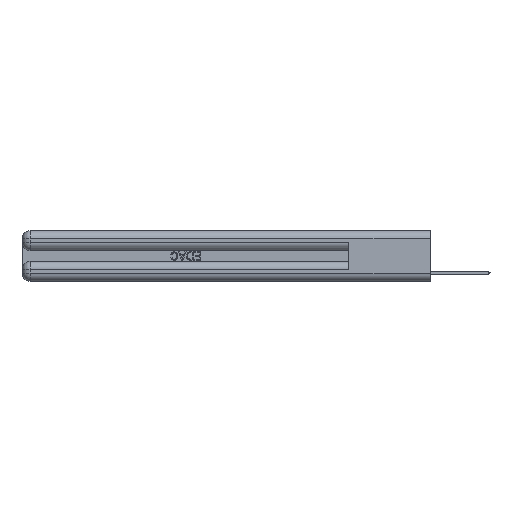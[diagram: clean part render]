
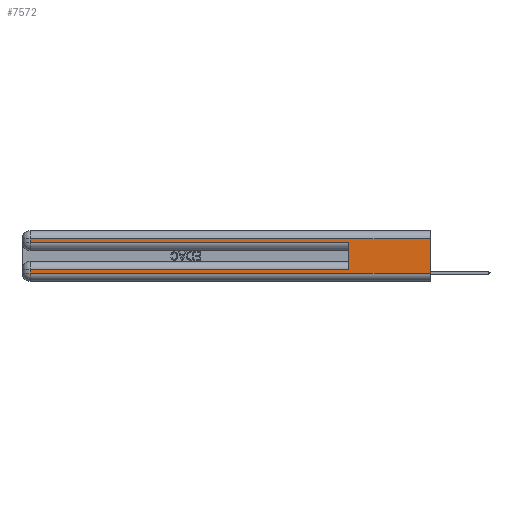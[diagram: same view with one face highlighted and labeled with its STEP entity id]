
A CAD part, left-side view. The second image highlights one B-rep face of the part: STEP entity #7572.
In plain terms, the highlighted planar face has unit normal (-1, 0, 0).
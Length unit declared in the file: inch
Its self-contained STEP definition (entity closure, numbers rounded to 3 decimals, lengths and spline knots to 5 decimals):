
#31 = CARTESIAN_POINT ( 'NONE',  ( 0., 2.94, 0.285 ) ) ;
#179 = CARTESIAN_POINT ( 'NONE',  ( 0., 2.94, 0.06 ) ) ;
#347 = VECTOR ( 'NONE', #25590, 39.37008 ) ;
#1287 = VERTEX_POINT ( 'NONE', #4405 ) ;
#1379 = ORIENTED_EDGE ( 'NONE', *, *, #2137, .F. ) ;
#1901 = DIRECTION ( 'NONE',  ( 0., 0., -1. ) ) ;
#2137 = EDGE_CURVE ( 'NONE', #29720, #19873, #12225, .T. ) ;
#2356 = CARTESIAN_POINT ( 'NONE',  ( 0., 2.94, 0.085 ) ) ;
#2806 = DIRECTION ( 'NONE',  ( 0., 1., 0. ) ) ;
#3886 = LINE ( 'NONE', #29007, #30766 ) ;
#4405 = CARTESIAN_POINT ( 'NONE',  ( 0., 2.94, 0.31 ) ) ;
#4489 = DIRECTION ( 'NONE',  ( 1., 0., 0. ) ) ;
#4772 = CARTESIAN_POINT ( 'NONE',  ( 0., 2.94, 0.37 ) ) ;
#5814 = EDGE_CURVE ( 'NONE', #18424, #19873, #11748, .T. ) ;
#6984 = LINE ( 'NONE', #7495, #13971 ) ;
#7495 = CARTESIAN_POINT ( 'NONE',  ( 0., 0., 0.085 ) ) ;
#7572 = ADVANCED_FACE ( 'NONE', ( #8146 ), #31122, .F. ) ;
#8146 = FACE_OUTER_BOUND ( 'NONE', #29288, .T. ) ;
#8517 = LINE ( 'NONE', #23102, #347 ) ;
#9180 = DIRECTION ( 'NONE',  ( 0., -1., 0. ) ) ;
#9893 = ORIENTED_EDGE ( 'NONE', *, *, #31795, .T. ) ;
#10034 = CARTESIAN_POINT ( 'NONE',  ( 0., 0., 0.31 ) ) ;
#10206 = VECTOR ( 'NONE', #9180, 39.37008 ) ;
#11000 = ORIENTED_EDGE ( 'NONE', *, *, #5814, .T. ) ;
#11731 = ORIENTED_EDGE ( 'NONE', *, *, #16184, .T. ) ;
#11748 = LINE ( 'NONE', #29020, #10206 ) ;
#12031 = CARTESIAN_POINT ( 'NONE',  ( 0., 0.6, 0.145 ) ) ;
#12225 = LINE ( 'NONE', #12031, #31355 ) ;
#12323 = EDGE_CURVE ( 'NONE', #23979, #31891, #14430, .T. ) ;
#13470 = CARTESIAN_POINT ( 'NONE',  ( 0., 0., 0.06 ) ) ;
#13510 = EDGE_CURVE ( 'NONE', #29037, #29497, #3886, .T. ) ;
#13971 = VECTOR ( 'NONE', #2806, 39.37008 ) ;
#14075 = LINE ( 'NONE', #13470, #25355 ) ;
#14430 = LINE ( 'NONE', #24626, #24527 ) ;
#16184 = EDGE_CURVE ( 'NONE', #1287, #18424, #27824, .T. ) ;
#17458 = DIRECTION ( 'NONE',  ( 0., 0., -1. ) ) ;
#18424 = VERTEX_POINT ( 'NONE', #31 ) ;
#19873 = VERTEX_POINT ( 'NONE', #26193 ) ;
#20364 = EDGE_CURVE ( 'NONE', #31891, #29497, #14075, .T. ) ;
#20964 = DIRECTION ( 'NONE',  ( 0., -1., 0. ) ) ;
#21144 = CARTESIAN_POINT ( 'NONE',  ( 0., 0., 0.37 ) ) ;
#21892 = ORIENTED_EDGE ( 'NONE', *, *, #13510, .F. ) ;
#21955 = VECTOR ( 'NONE', #17458, 39.37008 ) ;
#22322 = DIRECTION ( 'NONE',  ( 0., 0., 1. ) ) ;
#22791 = EDGE_CURVE ( 'NONE', #29037, #1287, #8517, .T. ) ;
#23102 = CARTESIAN_POINT ( 'NONE',  ( 0., 0., 0.31 ) ) ;
#23772 = CARTESIAN_POINT ( 'NONE',  ( 0., 0.6, 0.085 ) ) ;
#23979 = VERTEX_POINT ( 'NONE', #2356 ) ;
#24236 = DIRECTION ( 'NONE',  ( 0., 0., -1. ) ) ;
#24527 = VECTOR ( 'NONE', #24736, 39.37008 ) ;
#24626 = CARTESIAN_POINT ( 'NONE',  ( 0., 2.94, 0.37 ) ) ;
#24736 = DIRECTION ( 'NONE',  ( 0., 0., -1. ) ) ;
#25355 = VECTOR ( 'NONE', #20964, 39.37008 ) ;
#25538 = ORIENTED_EDGE ( 'NONE', *, *, #20364, .T. ) ;
#25590 = DIRECTION ( 'NONE',  ( 0., 1., 0. ) ) ;
#26193 = CARTESIAN_POINT ( 'NONE',  ( 0., 0.6, 0.285 ) ) ;
#27824 = LINE ( 'NONE', #4772, #21955 ) ;
#29007 = CARTESIAN_POINT ( 'NONE',  ( 0., 0., 0.37 ) ) ;
#29020 = CARTESIAN_POINT ( 'NONE',  ( 0., 0., 0.285 ) ) ;
#29037 = VERTEX_POINT ( 'NONE', #10034 ) ;
#29086 = CARTESIAN_POINT ( 'NONE',  ( 0., 0., 0.06 ) ) ;
#29288 = EDGE_LOOP ( 'NONE', ( #21892, #30101, #11731, #11000, #1379, #9893, #30371, #25538 ) ) ;
#29497 = VERTEX_POINT ( 'NONE', #29086 ) ;
#29720 = VERTEX_POINT ( 'NONE', #23772 ) ;
#30101 = ORIENTED_EDGE ( 'NONE', *, *, #22791, .T. ) ;
#30122 = AXIS2_PLACEMENT_3D ( 'NONE', #21144, #4489, #24236 ) ;
#30371 = ORIENTED_EDGE ( 'NONE', *, *, #12323, .T. ) ;
#30766 = VECTOR ( 'NONE', #1901, 39.37008 ) ;
#31122 = PLANE ( 'NONE',  #30122 ) ;
#31355 = VECTOR ( 'NONE', #22322, 39.37008 ) ;
#31795 = EDGE_CURVE ( 'NONE', #29720, #23979, #6984, .T. ) ;
#31891 = VERTEX_POINT ( 'NONE', #179 ) ;
